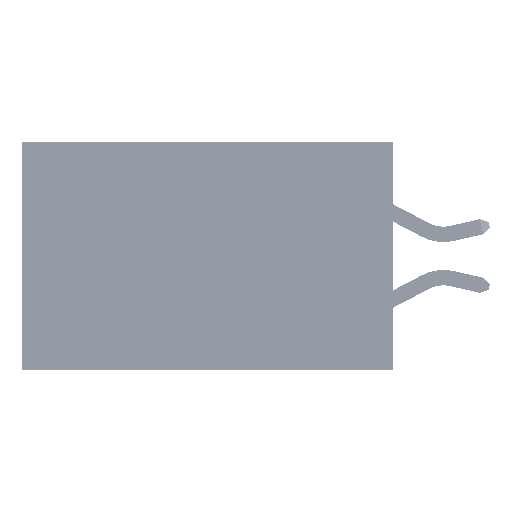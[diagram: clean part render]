
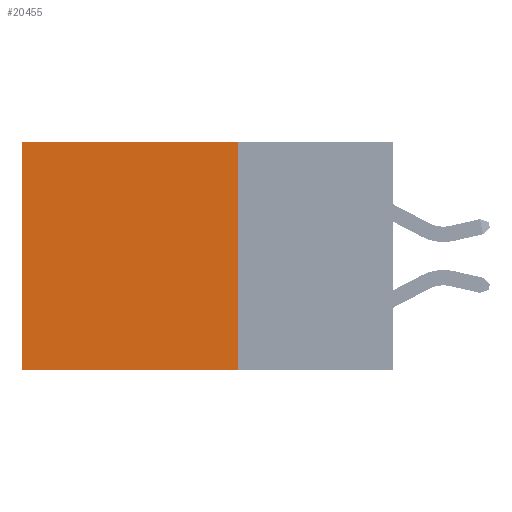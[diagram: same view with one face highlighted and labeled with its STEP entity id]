
A CAD part, left-side view. The second image highlights one B-rep face of the part: STEP entity #20455.
In plain terms, the highlighted planar face has unit normal (-1, 0, 0).
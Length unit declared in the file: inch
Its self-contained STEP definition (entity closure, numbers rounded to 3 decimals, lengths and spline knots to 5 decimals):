
#687 = EDGE_CURVE ( 'NONE', #43925, #15978, #32942, .T. ) ;
#1265 = CARTESIAN_POINT ( 'NONE',  ( 0.2875, 0.6, -0.37 ) ) ;
#3257 = CARTESIAN_POINT ( 'NONE',  ( 0.2875, 0.6, 0. ) ) ;
#5499 = AXIS2_PLACEMENT_3D ( 'NONE', #27775, #16381, #44320 ) ;
#8639 = ORIENTED_EDGE ( 'NONE', *, *, #687, .T. ) ;
#11028 = VECTOR ( 'NONE', #23610, 39.37008 ) ;
#11893 = ORIENTED_EDGE ( 'NONE', *, *, #46686, .F. ) ;
#12230 = FACE_OUTER_BOUND ( 'NONE', #27980, .T. ) ;
#12405 = VECTOR ( 'NONE', #28777, 39.37008 ) ;
#13251 = DIRECTION ( 'NONE',  ( 0., 0., -1. ) ) ;
#13267 = DIRECTION ( 'NONE',  ( 0., 1., 0. ) ) ;
#13494 = CARTESIAN_POINT ( 'NONE',  ( 0.2875, 0.6, 0. ) ) ;
#15978 = VERTEX_POINT ( 'NONE', #3257 ) ;
#16336 = ORIENTED_EDGE ( 'NONE', *, *, #22384, .T. ) ;
#16381 = DIRECTION ( 'NONE',  ( 1., 0., 0. ) ) ;
#16861 = LINE ( 'NONE', #21012, #12405 ) ;
#19757 = PLANE ( 'NONE',  #5499 ) ;
#20280 = CARTESIAN_POINT ( 'NONE',  ( 0.2875, 0.25, 0. ) ) ;
#20455 = ADVANCED_FACE ( 'NONE', ( #12230 ), #19757, .F. ) ;
#21012 = CARTESIAN_POINT ( 'NONE',  ( 0.2875, 0.25, -0.37 ) ) ;
#22384 = EDGE_CURVE ( 'NONE', #15978, #43656, #25430, .T. ) ;
#23610 = DIRECTION ( 'NONE',  ( 0., 0., -1. ) ) ;
#25430 = LINE ( 'NONE', #13494, #28640 ) ;
#27775 = CARTESIAN_POINT ( 'NONE',  ( 0.2875, 0.25, 0. ) ) ;
#27900 = EDGE_CURVE ( 'NONE', #35751, #43656, #16861, .T. ) ;
#27980 = EDGE_LOOP ( 'NONE', ( #16336, #44708, #11893, #8639 ) ) ;
#28640 = VECTOR ( 'NONE', #13251, 39.37008 ) ;
#28762 = CARTESIAN_POINT ( 'NONE',  ( 0.2875, 0.25, 0. ) ) ;
#28777 = DIRECTION ( 'NONE',  ( 0., 1., 0. ) ) ;
#32942 = LINE ( 'NONE', #20280, #37168 ) ;
#33798 = CARTESIAN_POINT ( 'NONE',  ( 0.2875, 0.25, -0.37 ) ) ;
#35751 = VERTEX_POINT ( 'NONE', #33798 ) ;
#37168 = VECTOR ( 'NONE', #13267, 39.37008 ) ;
#43656 = VERTEX_POINT ( 'NONE', #1265 ) ;
#43925 = VERTEX_POINT ( 'NONE', #46817 ) ;
#44320 = DIRECTION ( 'NONE',  ( 0., 0., -1. ) ) ;
#44708 = ORIENTED_EDGE ( 'NONE', *, *, #27900, .F. ) ;
#46686 = EDGE_CURVE ( 'NONE', #43925, #35751, #48188, .T. ) ;
#46817 = CARTESIAN_POINT ( 'NONE',  ( 0.2875, 0.25, 0. ) ) ;
#48188 = LINE ( 'NONE', #28762, #11028 ) ;
